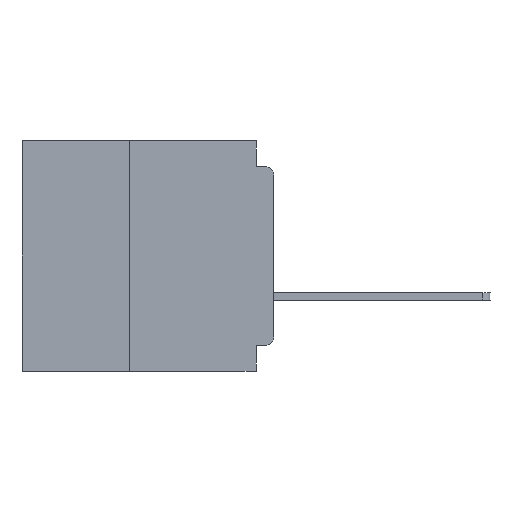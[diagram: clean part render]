
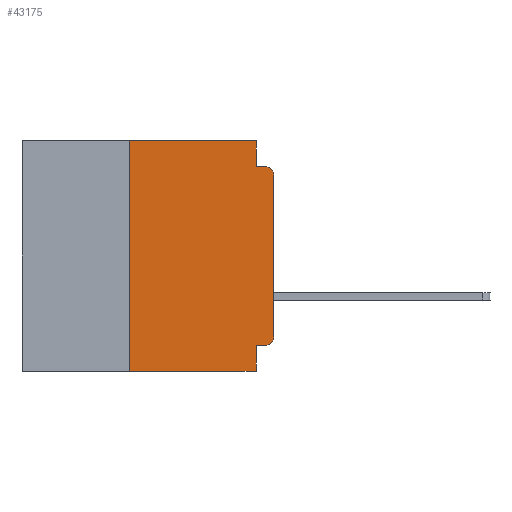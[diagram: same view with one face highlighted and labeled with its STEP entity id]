
A CAD part, left-side view. The second image highlights one B-rep face of the part: STEP entity #43175.
In plain terms, the highlighted planar face has unit normal (-1, 0, 0).
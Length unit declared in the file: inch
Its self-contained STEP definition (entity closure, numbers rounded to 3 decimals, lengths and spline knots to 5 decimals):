
#977 = VECTOR ( 'NONE', #24368, 39.37008 ) ;
#3374 = CARTESIAN_POINT ( 'NONE',  ( 0., 0.031, -0.4 ) ) ;
#6318 = CARTESIAN_POINT ( 'NONE',  ( 0., 0., -0.06 ) ) ;
#6352 = LINE ( 'NONE', #57878, #48389 ) ;
#7042 = DIRECTION ( 'NONE',  ( 0., 1., 0. ) ) ;
#7569 = CARTESIAN_POINT ( 'NONE',  ( 0., 0.031, 0. ) ) ;
#9019 = CARTESIAN_POINT ( 'NONE',  ( 0., 0.031, 0. ) ) ;
#9288 = VERTEX_POINT ( 'NONE', #20525 ) ;
#9642 = CARTESIAN_POINT ( 'NONE',  ( 0., 0.031, -0.355 ) ) ;
#10536 = DIRECTION ( 'NONE',  ( 0., -1., 0. ) ) ;
#11318 = ORIENTED_EDGE ( 'NONE', *, *, #45634, .F. ) ;
#12894 = VERTEX_POINT ( 'NONE', #9019 ) ;
#14226 = EDGE_CURVE ( 'NONE', #59410, #63788, #65502, .T. ) ;
#17615 = EDGE_CURVE ( 'NONE', #63788, #66359, #29915, .T. ) ;
#17827 = VECTOR ( 'NONE', #44124, 39.37008 ) ;
#17943 = LINE ( 'NONE', #66832, #31970 ) ;
#18437 = VERTEX_POINT ( 'NONE', #55303 ) ;
#18533 = EDGE_CURVE ( 'NONE', #51649, #18437, #52787, .T. ) ;
#20255 = EDGE_CURVE ( 'NONE', #53452, #59410, #35296, .T. ) ;
#20525 = CARTESIAN_POINT ( 'NONE',  ( 0., 0.031, -0.045 ) ) ;
#21760 = EDGE_CURVE ( 'NONE', #18437, #12894, #63069, .T. ) ;
#22361 = VECTOR ( 'NONE', #7042, 39.37008 ) ;
#22582 = PLANE ( 'NONE',  #51437 ) ;
#24302 = CARTESIAN_POINT ( 'NONE',  ( 0., 0.015, -0.34 ) ) ;
#24368 = DIRECTION ( 'NONE',  ( 0., 0., -1. ) ) ;
#24736 = DIRECTION ( 'NONE',  ( 0., 0., 1. ) ) ;
#25619 = ORIENTED_EDGE ( 'NONE', *, *, #60592, .F. ) ;
#27189 = CARTESIAN_POINT ( 'NONE',  ( 0., 0.015, -0.06 ) ) ;
#29597 = DIRECTION ( 'NONE',  ( 0., 0., -1. ) ) ;
#29915 = CIRCLE ( 'NONE', #55022, 0.015 ) ;
#30122 = DIRECTION ( 'NONE',  ( 0., -1., 0. ) ) ;
#31946 = FACE_OUTER_BOUND ( 'NONE', #37984, .T. ) ;
#31970 = VECTOR ( 'NONE', #30122, 39.37008 ) ;
#32483 = DIRECTION ( 'NONE',  ( 0., 0., -1. ) ) ;
#33170 = DIRECTION ( 'NONE',  ( 0., 0., -1. ) ) ;
#33489 = LINE ( 'NONE', #7569, #17827 ) ;
#34754 = LINE ( 'NONE', #54420, #22361 ) ;
#34936 = EDGE_CURVE ( 'NONE', #65990, #37676, #57062, .T. ) ;
#35296 = CIRCLE ( 'NONE', #62809, 0.015 ) ;
#35723 = CARTESIAN_POINT ( 'NONE',  ( 0., 0.25, -0.4 ) ) ;
#36466 = ORIENTED_EDGE ( 'NONE', *, *, #18533, .F. ) ;
#36813 = VECTOR ( 'NONE', #56406, 39.37008 ) ;
#37644 = VECTOR ( 'NONE', #58037, 39.37008 ) ;
#37676 = VERTEX_POINT ( 'NONE', #3374 ) ;
#37984 = EDGE_LOOP ( 'NONE', ( #43848, #51842, #45821, #25619, #63778, #36466, #40486, #41265, #11318, #38374 ) ) ;
#38374 = ORIENTED_EDGE ( 'NONE', *, *, #20255, .T. ) ;
#40486 = ORIENTED_EDGE ( 'NONE', *, *, #65415, .T. ) ;
#41265 = ORIENTED_EDGE ( 'NONE', *, *, #34936, .F. ) ;
#43175 = ADVANCED_FACE ( 'NONE', ( #31946 ), #22582, .F. ) ;
#43848 = ORIENTED_EDGE ( 'NONE', *, *, #14226, .T. ) ;
#44124 = DIRECTION ( 'NONE',  ( 0., 0., -1. ) ) ;
#45634 = EDGE_CURVE ( 'NONE', #53452, #65990, #34754, .T. ) ;
#45821 = ORIENTED_EDGE ( 'NONE', *, *, #65264, .F. ) ;
#46957 = CARTESIAN_POINT ( 'NONE',  ( 0., 0.015, -0.355 ) ) ;
#48389 = VECTOR ( 'NONE', #10536, 39.37008 ) ;
#50601 = CARTESIAN_POINT ( 'NONE',  ( 0., 0.031, -0.4 ) ) ;
#51174 = CARTESIAN_POINT ( 'NONE',  ( 0., 0.437, 0. ) ) ;
#51437 = AXIS2_PLACEMENT_3D ( 'NONE', #59307, #64578, #33170 ) ;
#51649 = VERTEX_POINT ( 'NONE', #35723 ) ;
#51842 = ORIENTED_EDGE ( 'NONE', *, *, #17615, .T. ) ;
#52776 = CARTESIAN_POINT ( 'NONE',  ( 0., 0., 0. ) ) ;
#52787 = LINE ( 'NONE', #66535, #65043 ) ;
#53452 = VERTEX_POINT ( 'NONE', #46957 ) ;
#54420 = CARTESIAN_POINT ( 'NONE',  ( 0., 0., -0.355 ) ) ;
#55022 = AXIS2_PLACEMENT_3D ( 'NONE', #27189, #63914, #32483 ) ;
#55062 = CARTESIAN_POINT ( 'NONE',  ( 0., 0.015, -0.045 ) ) ;
#55303 = CARTESIAN_POINT ( 'NONE',  ( 0., 0.25, 0. ) ) ;
#56406 = DIRECTION ( 'NONE',  ( 0., -1., 0. ) ) ;
#57062 = LINE ( 'NONE', #50601, #977 ) ;
#57878 = CARTESIAN_POINT ( 'NONE',  ( 0., 0.437, -0.4 ) ) ;
#58037 = DIRECTION ( 'NONE',  ( 0., 0., 1. ) ) ;
#59307 = CARTESIAN_POINT ( 'NONE',  ( 0., 0.437, 0. ) ) ;
#59410 = VERTEX_POINT ( 'NONE', #64977 ) ;
#60592 = EDGE_CURVE ( 'NONE', #12894, #9288, #33489, .T. ) ;
#61057 = DIRECTION ( 'NONE',  ( -1., 0., 0. ) ) ;
#62809 = AXIS2_PLACEMENT_3D ( 'NONE', #24302, #61057, #29597 ) ;
#63069 = LINE ( 'NONE', #51174, #36813 ) ;
#63778 = ORIENTED_EDGE ( 'NONE', *, *, #21760, .F. ) ;
#63788 = VERTEX_POINT ( 'NONE', #6318 ) ;
#63914 = DIRECTION ( 'NONE',  ( -1., 0., 0. ) ) ;
#64578 = DIRECTION ( 'NONE',  ( 1., 0., 0. ) ) ;
#64977 = CARTESIAN_POINT ( 'NONE',  ( 0., 0., -0.34 ) ) ;
#65043 = VECTOR ( 'NONE', #24736, 39.37008 ) ;
#65264 = EDGE_CURVE ( 'NONE', #9288, #66359, #17943, .T. ) ;
#65415 = EDGE_CURVE ( 'NONE', #51649, #37676, #6352, .T. ) ;
#65502 = LINE ( 'NONE', #52776, #37644 ) ;
#65990 = VERTEX_POINT ( 'NONE', #9642 ) ;
#66359 = VERTEX_POINT ( 'NONE', #55062 ) ;
#66535 = CARTESIAN_POINT ( 'NONE',  ( 0., 0.25, -0.4 ) ) ;
#66832 = CARTESIAN_POINT ( 'NONE',  ( 0., 0., -0.045 ) ) ;
